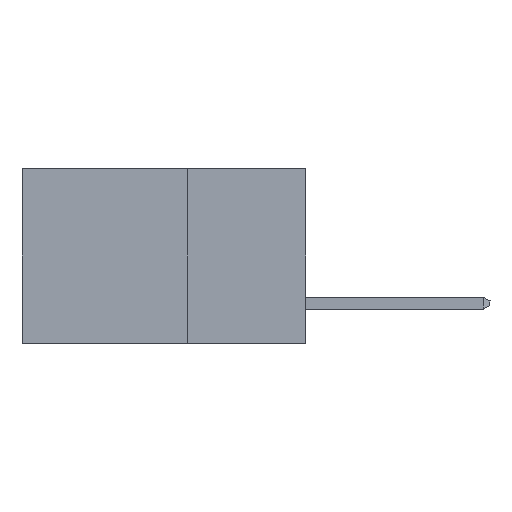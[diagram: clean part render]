
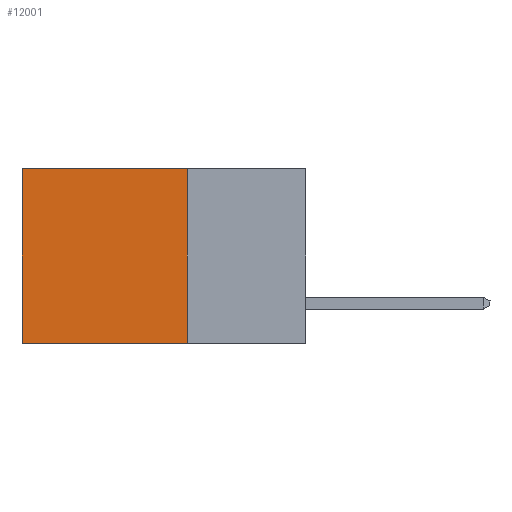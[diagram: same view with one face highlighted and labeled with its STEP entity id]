
A CAD part, left-side view. The second image highlights one B-rep face of the part: STEP entity #12001.
In plain terms, the highlighted planar face has unit normal (-1, 0, 0).
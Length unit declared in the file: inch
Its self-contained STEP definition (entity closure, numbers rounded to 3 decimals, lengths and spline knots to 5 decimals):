
#475 = VECTOR ( 'NONE', #7126, 39.37008 ) ;
#1132 = EDGE_CURVE ( 'NONE', #7127, #2902, #5093, .T. ) ;
#1573 = CARTESIAN_POINT ( 'NONE',  ( 0.298, 0.25, 0. ) ) ;
#2215 = EDGE_CURVE ( 'NONE', #2902, #9834, #13761, .T. ) ;
#2641 = CARTESIAN_POINT ( 'NONE',  ( 0.298, 0.6, 0. ) ) ;
#2902 = VERTEX_POINT ( 'NONE', #2641 ) ;
#2981 = VERTEX_POINT ( 'NONE', #12208 ) ;
#3240 = ORIENTED_EDGE ( 'NONE', *, *, #8262, .F. ) ;
#3610 = DIRECTION ( 'NONE',  ( 0., 0., -1. ) ) ;
#4606 = VECTOR ( 'NONE', #3610, 39.37008 ) ;
#4682 = CARTESIAN_POINT ( 'NONE',  ( 0.298, 0.6, 0. ) ) ;
#4773 = DIRECTION ( 'NONE',  ( 0., 0., -1. ) ) ;
#5093 = LINE ( 'NONE', #8804, #13508 ) ;
#5839 = CARTESIAN_POINT ( 'NONE',  ( 0.298, 0.25, 0. ) ) ;
#5861 = CARTESIAN_POINT ( 'NONE',  ( 0.298, 0.25, -0.37 ) ) ;
#5907 = CARTESIAN_POINT ( 'NONE',  ( 0.298, 0.6, -0.37 ) ) ;
#6355 = LINE ( 'NONE', #5839, #6543 ) ;
#6441 = PLANE ( 'NONE',  #14723 ) ;
#6543 = VECTOR ( 'NONE', #4773, 39.37008 ) ;
#6746 = ORIENTED_EDGE ( 'NONE', *, *, #1132, .T. ) ;
#7126 = DIRECTION ( 'NONE',  ( 0., 1., 0. ) ) ;
#7127 = VERTEX_POINT ( 'NONE', #13107 ) ;
#7137 = EDGE_CURVE ( 'NONE', #7127, #2981, #6355, .T. ) ;
#7395 = EDGE_LOOP ( 'NONE', ( #12805, #3240, #7760, #6746 ) ) ;
#7760 = ORIENTED_EDGE ( 'NONE', *, *, #7137, .F. ) ;
#8262 = EDGE_CURVE ( 'NONE', #2981, #9834, #13861, .T. ) ;
#8804 = CARTESIAN_POINT ( 'NONE',  ( 0.298, 0.25, 0. ) ) ;
#8983 = DIRECTION ( 'NONE',  ( 0., 0., -1. ) ) ;
#9834 = VERTEX_POINT ( 'NONE', #5907 ) ;
#10612 = FACE_OUTER_BOUND ( 'NONE', #7395, .T. ) ;
#12001 = ADVANCED_FACE ( 'NONE', ( #10612 ), #6441, .F. ) ;
#12208 = CARTESIAN_POINT ( 'NONE',  ( 0.298, 0.25, -0.37 ) ) ;
#12805 = ORIENTED_EDGE ( 'NONE', *, *, #2215, .T. ) ;
#13107 = CARTESIAN_POINT ( 'NONE',  ( 0.298, 0.25, 0. ) ) ;
#13508 = VECTOR ( 'NONE', #14863, 39.37008 ) ;
#13761 = LINE ( 'NONE', #4682, #4606 ) ;
#13814 = DIRECTION ( 'NONE',  ( 1., 0., 0. ) ) ;
#13861 = LINE ( 'NONE', #5861, #475 ) ;
#14723 = AXIS2_PLACEMENT_3D ( 'NONE', #1573, #13814, #8983 ) ;
#14863 = DIRECTION ( 'NONE',  ( 0., 1., 0. ) ) ;
